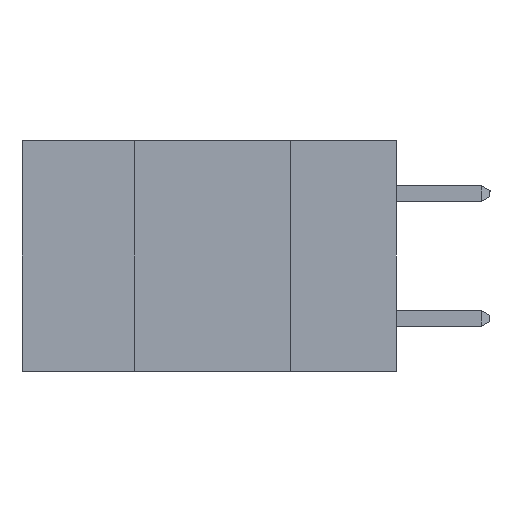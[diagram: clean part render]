
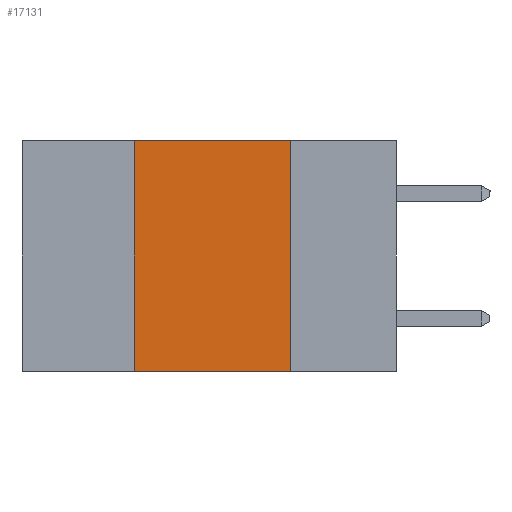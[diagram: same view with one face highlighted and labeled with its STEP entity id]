
A CAD part, left-side view. The second image highlights one B-rep face of the part: STEP entity #17131.
In plain terms, the highlighted planar face has unit normal (-1, 0, 0).
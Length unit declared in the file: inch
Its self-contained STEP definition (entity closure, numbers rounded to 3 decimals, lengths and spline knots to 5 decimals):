
#34 = VERTEX_POINT ( 'NONE', #14112 ) ;
#1039 = LINE ( 'NONE', #15880, #13012 ) ;
#1240 = ORIENTED_EDGE ( 'NONE', *, *, #3434, .F. ) ;
#1455 = CARTESIAN_POINT ( 'NONE',  ( 0., 0.17, -0.37 ) ) ;
#1622 = LINE ( 'NONE', #18065, #4585 ) ;
#1655 = ORIENTED_EDGE ( 'NONE', *, *, #6681, .F. ) ;
#2252 = DIRECTION ( 'NONE',  ( 0., 0., 1. ) ) ;
#2852 = DIRECTION ( 'NONE',  ( 0., -1., 0. ) ) ;
#2944 = ORIENTED_EDGE ( 'NONE', *, *, #18392, .T. ) ;
#3434 = EDGE_CURVE ( 'NONE', #16713, #11493, #12722, .T. ) ;
#4585 = VECTOR ( 'NONE', #2852, 39.37008 ) ;
#4602 = VECTOR ( 'NONE', #14611, 39.37008 ) ;
#5185 = VERTEX_POINT ( 'NONE', #16830 ) ;
#6681 = EDGE_CURVE ( 'NONE', #5185, #34, #1039, .T. ) ;
#7048 = CARTESIAN_POINT ( 'NONE',  ( 0., 0.6, -0.37 ) ) ;
#7371 = VECTOR ( 'NONE', #14712, 39.37008 ) ;
#8245 = CARTESIAN_POINT ( 'NONE',  ( 0., 0.17, -0.37 ) ) ;
#8559 = LINE ( 'NONE', #7048, #7371 ) ;
#10633 = DIRECTION ( 'NONE',  ( 0., 0., -1. ) ) ;
#11493 = VERTEX_POINT ( 'NONE', #1455 ) ;
#11830 = EDGE_CURVE ( 'NONE', #34, #16713, #1622, .T. ) ;
#12426 = AXIS2_PLACEMENT_3D ( 'NONE', #18196, #16893, #10633 ) ;
#12722 = LINE ( 'NONE', #8245, #4602 ) ;
#13012 = VECTOR ( 'NONE', #2252, 39.37008 ) ;
#14112 = CARTESIAN_POINT ( 'NONE',  ( 0., 0.42, 0. ) ) ;
#14611 = DIRECTION ( 'NONE',  ( 0., 0., -1. ) ) ;
#14615 = PLANE ( 'NONE',  #12426 ) ;
#14712 = DIRECTION ( 'NONE',  ( 0., -1., 0. ) ) ;
#15007 = FACE_OUTER_BOUND ( 'NONE', #17400, .T. ) ;
#15421 = CARTESIAN_POINT ( 'NONE',  ( 0., 0.17, 0. ) ) ;
#15880 = CARTESIAN_POINT ( 'NONE',  ( 0., 0.42, -0.37 ) ) ;
#16080 = ORIENTED_EDGE ( 'NONE', *, *, #11830, .F. ) ;
#16713 = VERTEX_POINT ( 'NONE', #15421 ) ;
#16830 = CARTESIAN_POINT ( 'NONE',  ( 0., 0.42, -0.37 ) ) ;
#16893 = DIRECTION ( 'NONE',  ( 1., 0., 0. ) ) ;
#17131 = ADVANCED_FACE ( 'NONE', ( #15007 ), #14615, .F. ) ;
#17400 = EDGE_LOOP ( 'NONE', ( #1240, #16080, #1655, #2944 ) ) ;
#18065 = CARTESIAN_POINT ( 'NONE',  ( 0., 0.6, 0. ) ) ;
#18196 = CARTESIAN_POINT ( 'NONE',  ( 0., 0.6, 0. ) ) ;
#18392 = EDGE_CURVE ( 'NONE', #5185, #11493, #8559, .T. ) ;
